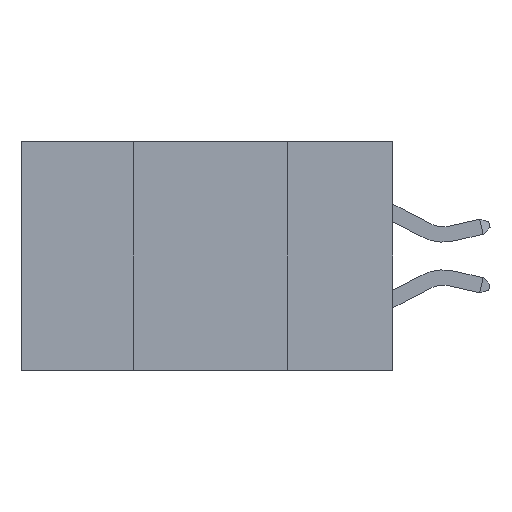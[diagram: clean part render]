
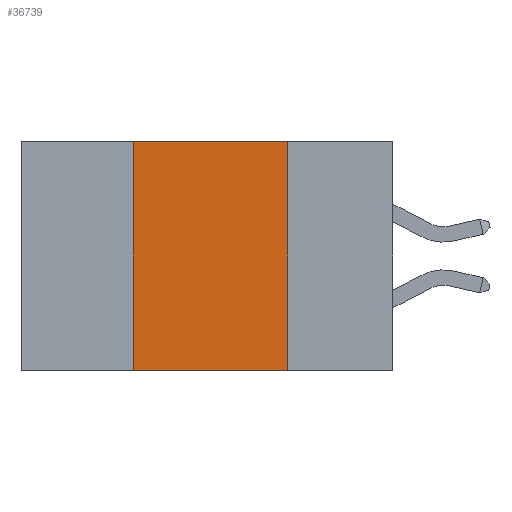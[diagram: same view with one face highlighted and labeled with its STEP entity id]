
A CAD part, left-side view. The second image highlights one B-rep face of the part: STEP entity #36739.
In plain terms, the highlighted planar face has unit normal (-1, 0, 0).
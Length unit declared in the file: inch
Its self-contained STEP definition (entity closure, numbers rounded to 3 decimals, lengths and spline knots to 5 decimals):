
#1474 = CARTESIAN_POINT ( 'NONE',  ( 0., 0.17, 0. ) ) ;
#1826 = DIRECTION ( 'NONE',  ( 0., 0., -1. ) ) ;
#2250 = LINE ( 'NONE', #7692, #31820 ) ;
#4003 = CARTESIAN_POINT ( 'NONE',  ( 0., 0.17, -0.37 ) ) ;
#5193 = VERTEX_POINT ( 'NONE', #15398 ) ;
#7658 = CARTESIAN_POINT ( 'NONE',  ( 0., 0.6, 0. ) ) ;
#7692 = CARTESIAN_POINT ( 'NONE',  ( 0., 0.17, 0. ) ) ;
#7699 = CARTESIAN_POINT ( 'NONE',  ( 0., 0.42, -0.37 ) ) ;
#7845 = VERTEX_POINT ( 'NONE', #4003 ) ;
#9570 = ORIENTED_EDGE ( 'NONE', *, *, #26986, .F. ) ;
#9719 = ORIENTED_EDGE ( 'NONE', *, *, #11343, .F. ) ;
#9770 = EDGE_CURVE ( 'NONE', #28942, #7845, #14290, .T. ) ;
#10033 = PLANE ( 'NONE',  #16540 ) ;
#10382 = ORIENTED_EDGE ( 'NONE', *, *, #14787, .F. ) ;
#11343 = EDGE_CURVE ( 'NONE', #5193, #28263, #33500, .T. ) ;
#11499 = VECTOR ( 'NONE', #30818, 39.37008 ) ;
#13206 = DIRECTION ( 'NONE',  ( 0., 0., -1. ) ) ;
#14290 = LINE ( 'NONE', #18037, #19223 ) ;
#14787 = EDGE_CURVE ( 'NONE', #28942, #5193, #33883, .T. ) ;
#15398 = CARTESIAN_POINT ( 'NONE',  ( 0., 0.42, 0. ) ) ;
#16540 = AXIS2_PLACEMENT_3D ( 'NONE', #7658, #21866, #13206 ) ;
#17508 = DIRECTION ( 'NONE',  ( 0., 0., 1. ) ) ;
#18037 = CARTESIAN_POINT ( 'NONE',  ( 0., 0.6, -0.37 ) ) ;
#19223 = VECTOR ( 'NONE', #35286, 39.37008 ) ;
#21866 = DIRECTION ( 'NONE',  ( 1., 0., 0. ) ) ;
#24602 = ORIENTED_EDGE ( 'NONE', *, *, #9770, .T. ) ;
#25856 = FACE_OUTER_BOUND ( 'NONE', #30763, .T. ) ;
#26986 = EDGE_CURVE ( 'NONE', #28263, #7845, #2250, .T. ) ;
#28263 = VERTEX_POINT ( 'NONE', #1474 ) ;
#28942 = VERTEX_POINT ( 'NONE', #7699 ) ;
#30763 = EDGE_LOOP ( 'NONE', ( #9570, #9719, #10382, #24602 ) ) ;
#30818 = DIRECTION ( 'NONE',  ( 0., -1., 0. ) ) ;
#31820 = VECTOR ( 'NONE', #1826, 39.37008 ) ;
#33219 = CARTESIAN_POINT ( 'NONE',  ( 0., 0.6, 0. ) ) ;
#33500 = LINE ( 'NONE', #33219, #11499 ) ;
#33883 = LINE ( 'NONE', #36420, #35636 ) ;
#35286 = DIRECTION ( 'NONE',  ( 0., -1., 0. ) ) ;
#35636 = VECTOR ( 'NONE', #17508, 39.37008 ) ;
#36420 = CARTESIAN_POINT ( 'NONE',  ( 0., 0.42, 0. ) ) ;
#36739 = ADVANCED_FACE ( 'NONE', ( #25856 ), #10033, .F. ) ;
